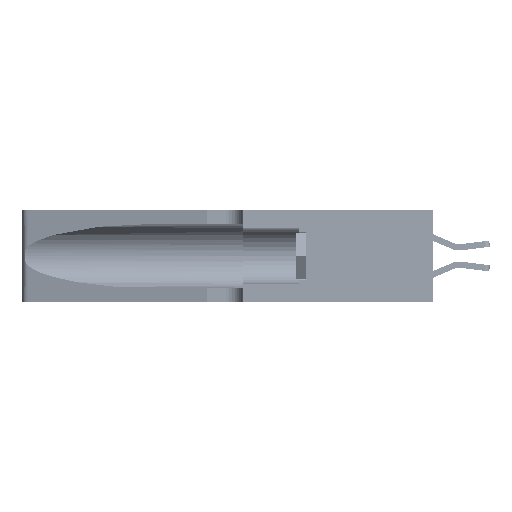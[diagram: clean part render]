
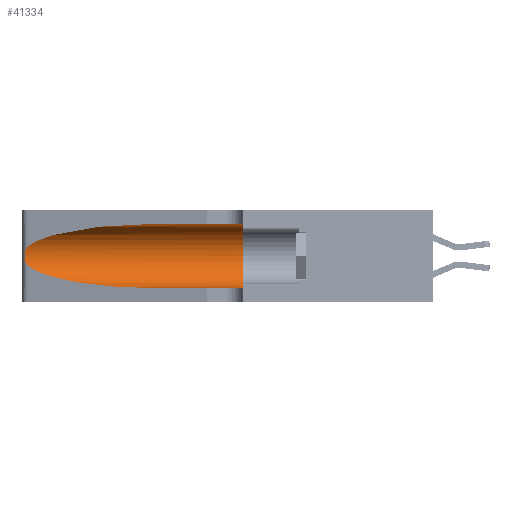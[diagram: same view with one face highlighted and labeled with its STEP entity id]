
A CAD part, left-side view. The second image highlights one B-rep face of the part: STEP entity #41334.
In plain terms, the highlighted cylindrical face has radius 3.308 mm (diameter 6.617 mm), a partial arc.
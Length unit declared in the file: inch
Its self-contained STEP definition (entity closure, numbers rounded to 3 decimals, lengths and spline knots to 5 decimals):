
#306 = CARTESIAN_POINT ( 'NONE',  ( 0.1305, 1.61858, 0.31525 ) ) ;
#2586 = B_SPLINE_CURVE_WITH_KNOTS ( 'NONE', 3,
 ( #14023, #22156, #13845, #35331, #18098, #26433, #52146, #18454, #5286, #47680, #22518, #22341, #6022, #18269 ),
 .UNSPECIFIED., .F., .F.,
 ( 4, 2, 2, 2, 2, 2, 4 ),
 ( 0., 0.00027, 0.00053, 0.00107, 0.0016, 0.00187, 0.00214 ),
 .UNSPECIFIED. ) ;
#3461 = CARTESIAN_POINT ( 'NONE',  ( 0.18966, 0.96281, 0.05475 ) ) ;
#4573 = AXIS2_PLACEMENT_3D ( 'NONE', #24420, #40764, #20140 ) ;
#4895 = CARTESIAN_POINT ( 'NONE',  ( 0.25487, 1.22718, 0.22369 ) ) ;
#5286 = CARTESIAN_POINT ( 'NONE',  ( 0.26017, 1.23833, 0.17102 ) ) ;
#5577 = CARTESIAN_POINT ( 'NONE',  ( 0.1305, 1.61858, 0.185 ) ) ;
#6022 = CARTESIAN_POINT ( 'NONE',  ( 0.25555, 1.22993, 0.14849 ) ) ;
#9332 = DIRECTION ( 'NONE',  ( 0., -1., 0. ) ) ;
#9907 = VERTEX_POINT ( 'NONE', #49286 ) ;
#10388 = VERTEX_POINT ( 'NONE', #47781 ) ;
#11047 = LINE ( 'NONE', #306, #54940 ) ;
#11911 = VERTEX_POINT ( 'NONE', #15082 ) ;
#13490 = ORIENTED_EDGE ( 'NONE', *, *, #29336, .F. ) ;
#13845 = CARTESIAN_POINT ( 'NONE',  ( 0.25639, 1.23184, 0.21858 ) ) ;
#14023 = CARTESIAN_POINT ( 'NONE',  ( 0.25487, 1.22718, 0.22369 ) ) ;
#15082 = CARTESIAN_POINT ( 'NONE',  ( 0.1305, 0.72297, 0.05475 ) ) ;
#17719 = CARTESIAN_POINT ( 'NONE',  ( 0.1305, 0.72297, 0.31525 ) ) ;
#18098 = CARTESIAN_POINT ( 'NONE',  ( 0.25854, 1.2359, 0.20912 ) ) ;
#18269 = CARTESIAN_POINT ( 'NONE',  ( 0.25487, 1.22718, 0.14631 ) ) ;
#18454 = CARTESIAN_POINT ( 'NONE',  ( 0.26075, 1.23896, 0.178 ) ) ;
#18573 = AXIS2_PLACEMENT_3D ( 'NONE', #5577, #30629, #34714 ) ;
#19291 = VECTOR ( 'NONE', #9332, 39.37008 ) ;
#19653 = CARTESIAN_POINT ( 'NONE',  ( 0.1305, 0.72297, 0.31525 ) ) ;
#19712 = EDGE_CURVE ( 'NONE', #37946, #11911, #41078, .T. ) ;
#20140 = DIRECTION ( 'NONE',  ( 0., 0., 1. ) ) ;
#20787 = EDGE_CURVE ( 'NONE', #29992, #32660, #40366, .T. ) ;
#22156 = CARTESIAN_POINT ( 'NONE',  ( 0.25555, 1.22994, 0.2215 ) ) ;
#22341 = CARTESIAN_POINT ( 'NONE',  ( 0.25639, 1.23186, 0.15144 ) ) ;
#22518 = CARTESIAN_POINT ( 'NONE',  ( 0.25789, 1.23486, 0.15765 ) ) ;
#22639 = ORIENTED_EDGE ( 'NONE', *, *, #25834, .T. ) ;
#23750 = CARTESIAN_POINT ( 'NONE',  ( 0.18966, 0.96281, 0.31525 ) ) ;
#24217 = ORIENTED_EDGE ( 'NONE', *, *, #19712, .T. ) ;
#24420 = CARTESIAN_POINT ( 'NONE',  ( 0.1305, 0.35, 0.185 ) ) ;
#25656 = ORIENTED_EDGE ( 'NONE', *, *, #20787, .T. ) ;
#25834 = EDGE_CURVE ( 'NONE', #11911, #10388, #30593, .T. ) ;
#26433 = CARTESIAN_POINT ( 'NONE',  ( 0.26018, 1.23835, 0.19895 ) ) ;
#27074 = ORIENTED_EDGE ( 'NONE', *, *, #52973, .T. ) ;
#29336 = EDGE_CURVE ( 'NONE', #29992, #9907, #11047, .T. ) ;
#29622 = FACE_OUTER_BOUND ( 'NONE', #51648, .T. ) ;
#29992 = VERTEX_POINT ( 'NONE', #17719 ) ;
#30593 = LINE ( 'NONE', #52073, #19291 ) ;
#30629 = DIRECTION ( 'NONE',  ( 0., -1., 0. ) ) ;
#32225 = CARTESIAN_POINT ( 'NONE',  ( 0.25487, 1.22718, 0.14631 ) ) ;
#32660 = VERTEX_POINT ( 'NONE', #4895 ) ;
#34714 = DIRECTION ( 'NONE',  ( 0., 0., -1. ) ) ;
#35331 = CARTESIAN_POINT ( 'NONE',  ( 0.25787, 1.23484, 0.2124 ) ) ;
#35443 = ORIENTED_EDGE ( 'NONE', *, *, #37955, .F. ) ;
#35570 = CYLINDRICAL_SURFACE ( 'NONE', #18573, 0.13025 ) ;
#35999 = CARTESIAN_POINT ( 'NONE',  ( 0.25487, 1.22718, 0.22369 ) ) ;
#36627 = CIRCLE ( 'NONE', #4573, 0.13025 ) ;
#37946 = VERTEX_POINT ( 'NONE', #32225 ) ;
#37955 = EDGE_CURVE ( 'NONE', #9907, #10388, #36627, .T. ) ;
#40366 =( BOUNDED_CURVE ( )  B_SPLINE_CURVE ( 3, ( #19653, #23750, #52998, #35999 ),
 .UNSPECIFIED., .F., .F. ) 
 B_SPLINE_CURVE_WITH_KNOTS ( ( 4, 4 ),
 ( 1.5708, 2.84003 ),
 .UNSPECIFIED. ) 
 CURVE ( )  GEOMETRIC_REPRESENTATION_ITEM ( )  RATIONAL_B_SPLINE_CURVE ( ( 1., 0.87, 0.87, 1. ) ) 
 REPRESENTATION_ITEM ( '' )  );
#40764 = DIRECTION ( 'NONE',  ( 0., 1., 0. ) ) ;
#41078 =( BOUNDED_CURVE ( )  B_SPLINE_CURVE ( 3, ( #45828, #54431, #3461, #46393 ),
 .UNSPECIFIED., .F., .F. ) 
 B_SPLINE_CURVE_WITH_KNOTS ( ( 4, 4 ),
 ( 3.44316, 4.71239 ),
 .UNSPECIFIED. ) 
 CURVE ( )  GEOMETRIC_REPRESENTATION_ITEM ( )  RATIONAL_B_SPLINE_CURVE ( ( 1., 0.87, 0.87, 1. ) ) 
 REPRESENTATION_ITEM ( '' )  );
#41334 = ADVANCED_FACE ( 'NONE', ( #29622 ), #35570, .F. ) ;
#45828 = CARTESIAN_POINT ( 'NONE',  ( 0.25487, 1.22718, 0.14631 ) ) ;
#46393 = CARTESIAN_POINT ( 'NONE',  ( 0.1305, 0.72297, 0.05475 ) ) ;
#47547 = DIRECTION ( 'NONE',  ( 0., -1., 0. ) ) ;
#47680 = CARTESIAN_POINT ( 'NONE',  ( 0.25856, 1.23593, 0.16098 ) ) ;
#47781 = CARTESIAN_POINT ( 'NONE',  ( 0.1305, 0.35, 0.05475 ) ) ;
#49286 = CARTESIAN_POINT ( 'NONE',  ( 0.1305, 0.35, 0.31525 ) ) ;
#51648 = EDGE_LOOP ( 'NONE', ( #25656, #27074, #24217, #22639, #35443, #13490 ) ) ;
#52073 = CARTESIAN_POINT ( 'NONE',  ( 0.1305, 1.61858, 0.05475 ) ) ;
#52146 = CARTESIAN_POINT ( 'NONE',  ( 0.26075, 1.23896, 0.19203 ) ) ;
#52973 = EDGE_CURVE ( 'NONE', #32660, #37946, #2586, .T. ) ;
#52998 = CARTESIAN_POINT ( 'NONE',  ( 0.2373, 1.15595, 0.28018 ) ) ;
#54431 = CARTESIAN_POINT ( 'NONE',  ( 0.2373, 1.15595, 0.08982 ) ) ;
#54940 = VECTOR ( 'NONE', #47547, 39.37008 ) ;
